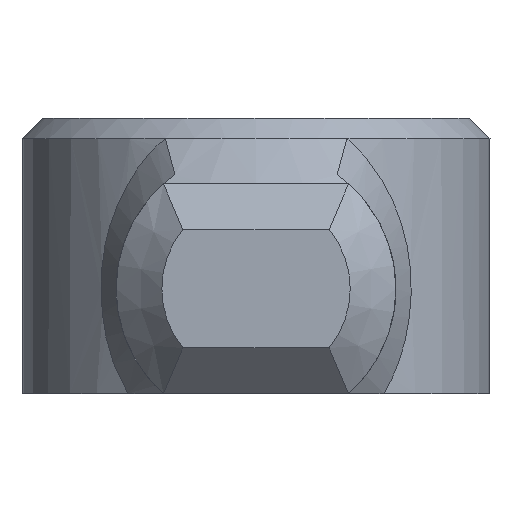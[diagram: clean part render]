
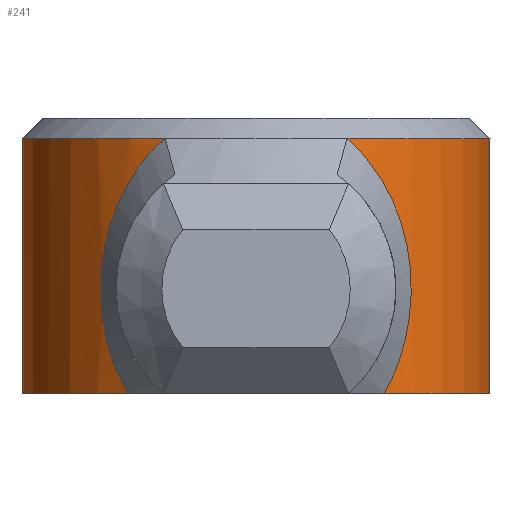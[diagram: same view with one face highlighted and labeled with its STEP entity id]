
A CAD part, left-side view. The second image highlights one B-rep face of the part: STEP entity #241.
In plain terms, the highlighted cylindrical face has radius 4.25 mm (diameter 8.501 mm), a partial arc.
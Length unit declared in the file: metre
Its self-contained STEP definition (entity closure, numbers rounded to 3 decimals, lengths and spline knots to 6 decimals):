
#18=CYLINDRICAL_SURFACE('',#273,0.004251);
#24=B_SPLINE_CURVE_WITH_KNOTS('',3,(#382,#383,#384,#385,#386,#387,#388,
#389),.UNSPECIFIED.,.F.,.F.,(4,1,1,1,1,4),(0.,0.25,0.5,0.625,0.75,1.),
 .UNSPECIFIED.);
#25=B_SPLINE_CURVE_WITH_KNOTS('',3,(#393,#394,#395,#396,#397,#398,#399,
#400,#401),.UNSPECIFIED.,.F.,.F.,(4,1,1,1,1,1,4),(0.,0.25,0.375,0.5,0.625,
0.75,1.),.UNSPECIFIED.);
#66=ORIENTED_EDGE('',*,*,#136,.T.);
#67=ORIENTED_EDGE('',*,*,#137,.T.);
#68=ORIENTED_EDGE('',*,*,#138,.T.);
#69=ORIENTED_EDGE('',*,*,#130,.T.);
#130=EDGE_CURVE('',#166,#165,#184,.T.);
#136=EDGE_CURVE('',#165,#171,#24,.T.);
#137=EDGE_CURVE('',#171,#172,#186,.T.);
#138=EDGE_CURVE('',#172,#166,#25,.T.);
#165=VERTEX_POINT('',#365);
#166=VERTEX_POINT('',#367);
#171=VERTEX_POINT('',#390);
#172=VERTEX_POINT('',#392);
#184=CIRCLE('',#270,0.004251);
#186=CIRCLE('',#274,0.004251);
#196=EDGE_LOOP('',(#66,#67,#68,#69));
#216=FACE_BOUND('',#196,.T.);
#241=ADVANCED_FACE('',(#216),#18,.T.);
#270=AXIS2_PLACEMENT_3D('',#366,#301,#302);
#273=AXIS2_PLACEMENT_3D('',#381,#310,#311);
#274=AXIS2_PLACEMENT_3D('',#391,#312,#313);
#301=DIRECTION('',(0.,0.,1.));
#302=DIRECTION('',(1.,0.,0.));
#310=DIRECTION('',(0.,0.,-1.));
#311=DIRECTION('',(-1.,0.,0.));
#312=DIRECTION('',(0.,0.,-1.));
#313=DIRECTION('',(-1.,0.,0.));
#365=CARTESIAN_POINT('',(-0.014039,0.002326,0.022479));
#366=CARTESIAN_POINT('',(-0.010481,0.,0.022479));
#367=CARTESIAN_POINT('',(-0.01404,-0.002325,0.022479));
#381=CARTESIAN_POINT('',(-0.010481,0.,0.026289));
#382=CARTESIAN_POINT('',(-0.014039,0.002326,0.022479));
#383=CARTESIAN_POINT('',(-0.013899,0.00254,0.022853));
#384=CARTESIAN_POINT('',(-0.013663,0.002821,0.023609));
#385=CARTESIAN_POINT('',(-0.013649,0.002836,0.024815));
#386=CARTESIAN_POINT('',(-0.013813,0.002644,0.025617));
#387=CARTESIAN_POINT('',(-0.014068,0.002301,0.026422));
#388=CARTESIAN_POINT('',(-0.014274,0.001946,0.026861));
#389=CARTESIAN_POINT('',(-0.0144,0.001647,0.027119));
#390=CARTESIAN_POINT('',(-0.0144,0.001647,0.027117));
#391=CARTESIAN_POINT('',(-0.010481,0.,0.027111));
#392=CARTESIAN_POINT('',(-0.014398,-0.001652,0.027115));
#393=CARTESIAN_POINT('',(-0.0144,-0.001647,0.027119));
#394=CARTESIAN_POINT('',(-0.014276,-0.001942,0.026865));
#395=CARTESIAN_POINT('',(-0.01407,-0.002298,0.026421));
#396=CARTESIAN_POINT('',(-0.013813,-0.002644,0.025617));
#397=CARTESIAN_POINT('',(-0.013692,-0.002786,0.025012));
#398=CARTESIAN_POINT('',(-0.013645,-0.002839,0.024336));
#399=CARTESIAN_POINT('',(-0.013729,-0.002744,0.023421));
#400=CARTESIAN_POINT('',(-0.013899,-0.002541,0.022855));
#401=CARTESIAN_POINT('',(-0.01404,-0.002325,0.022479));
